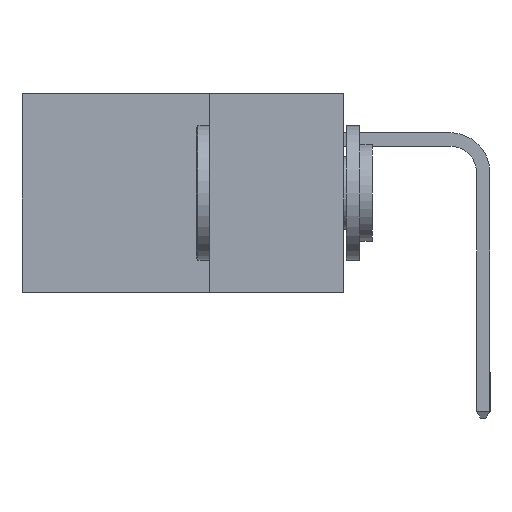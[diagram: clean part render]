
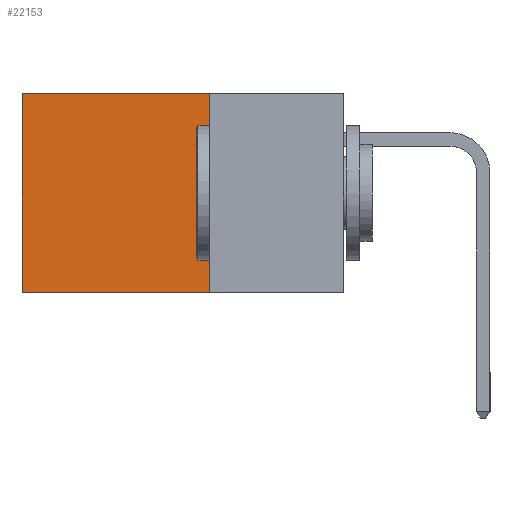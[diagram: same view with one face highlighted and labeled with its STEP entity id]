
A CAD part, left-side view. The second image highlights one B-rep face of the part: STEP entity #22153.
In plain terms, the highlighted planar face has unit normal (-1, 0, 0).
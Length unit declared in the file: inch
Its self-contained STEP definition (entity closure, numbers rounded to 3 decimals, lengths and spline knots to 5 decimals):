
#1945 = DIRECTION ( 'NONE',  ( 0., 1., 0. ) ) ;
#2404 = DIRECTION ( 'NONE',  ( 1., 0., 0. ) ) ;
#2438 = DIRECTION ( 'NONE',  ( 0., 0., -1. ) ) ;
#4056 = LINE ( 'NONE', #13920, #18042 ) ;
#7458 = VERTEX_POINT ( 'NONE', #25448 ) ;
#8908 = ORIENTED_EDGE ( 'NONE', *, *, #21546, .T. ) ;
#9056 = PLANE ( 'NONE',  #12389 ) ;
#9386 = CARTESIAN_POINT ( 'NONE',  ( 0.298, 0.6, 0. ) ) ;
#11398 = CARTESIAN_POINT ( 'NONE',  ( 0.298, 0.25, 0. ) ) ;
#12019 = LINE ( 'NONE', #25809, #16565 ) ;
#12332 = VECTOR ( 'NONE', #16843, 39.37008 ) ;
#12389 = AXIS2_PLACEMENT_3D ( 'NONE', #11398, #2404, #24655 ) ;
#13920 = CARTESIAN_POINT ( 'NONE',  ( 0.298, 0.25, 0. ) ) ;
#15259 = ORIENTED_EDGE ( 'NONE', *, *, #22886, .F. ) ;
#15454 = EDGE_CURVE ( 'NONE', #7458, #24840, #4056, .T. ) ;
#15468 = VERTEX_POINT ( 'NONE', #9386 ) ;
#16012 = VERTEX_POINT ( 'NONE', #24383 ) ;
#16565 = VECTOR ( 'NONE', #28224, 39.37008 ) ;
#16647 = CARTESIAN_POINT ( 'NONE',  ( 0.298, 0.25, -0.37 ) ) ;
#16843 = DIRECTION ( 'NONE',  ( 0., 1., 0. ) ) ;
#17744 = EDGE_LOOP ( 'NONE', ( #25935, #15259, #22292, #8908 ) ) ;
#18042 = VECTOR ( 'NONE', #2438, 39.37008 ) ;
#18472 = VECTOR ( 'NONE', #1945, 39.37008 ) ;
#18892 = EDGE_CURVE ( 'NONE', #15468, #16012, #12019, .T. ) ;
#21546 = EDGE_CURVE ( 'NONE', #7458, #15468, #28895, .T. ) ;
#22153 = ADVANCED_FACE ( 'NONE', ( #28501 ), #9056, .F. ) ;
#22292 = ORIENTED_EDGE ( 'NONE', *, *, #15454, .F. ) ;
#22758 = LINE ( 'NONE', #16647, #12332 ) ;
#22886 = EDGE_CURVE ( 'NONE', #24840, #16012, #22758, .T. ) ;
#23350 = CARTESIAN_POINT ( 'NONE',  ( 0.298, 0.25, -0.37 ) ) ;
#24383 = CARTESIAN_POINT ( 'NONE',  ( 0.298, 0.6, -0.37 ) ) ;
#24394 = CARTESIAN_POINT ( 'NONE',  ( 0.298, 0.25, 0. ) ) ;
#24655 = DIRECTION ( 'NONE',  ( 0., 0., -1. ) ) ;
#24840 = VERTEX_POINT ( 'NONE', #23350 ) ;
#25448 = CARTESIAN_POINT ( 'NONE',  ( 0.298, 0.25, 0. ) ) ;
#25809 = CARTESIAN_POINT ( 'NONE',  ( 0.298, 0.6, 0. ) ) ;
#25935 = ORIENTED_EDGE ( 'NONE', *, *, #18892, .T. ) ;
#28224 = DIRECTION ( 'NONE',  ( 0., 0., -1. ) ) ;
#28501 = FACE_OUTER_BOUND ( 'NONE', #17744, .T. ) ;
#28895 = LINE ( 'NONE', #24394, #18472 ) ;
